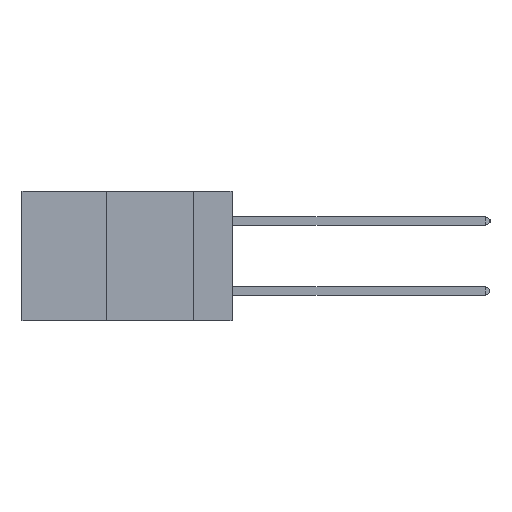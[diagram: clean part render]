
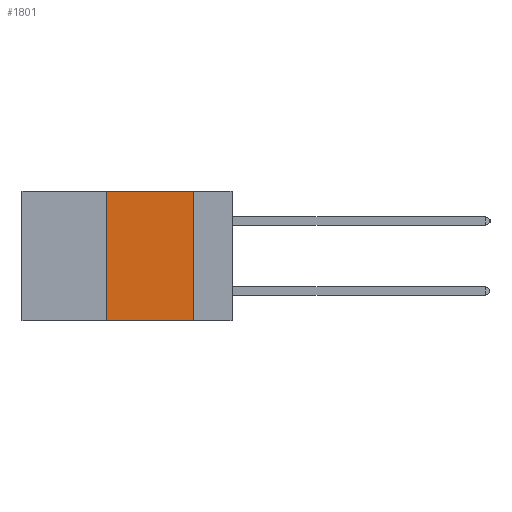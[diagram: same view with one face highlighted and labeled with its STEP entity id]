
A CAD part, left-side view. The second image highlights one B-rep face of the part: STEP entity #1801.
In plain terms, the highlighted planar face has unit normal (-1, 0, 0).
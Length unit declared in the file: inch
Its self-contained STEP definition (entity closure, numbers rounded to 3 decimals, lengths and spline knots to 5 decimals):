
#631 = EDGE_CURVE ( 'NONE', #7029, #7273, #1548, .T. ) ;
#1147 = EDGE_CURVE ( 'NONE', #3780, #7273, #8352, .T. ) ;
#1320 = PLANE ( 'NONE',  #10939 ) ;
#1548 = LINE ( 'NONE', #11987, #9646 ) ;
#1607 = DIRECTION ( 'NONE',  ( 0., 0., 1. ) ) ;
#1782 = EDGE_CURVE ( 'NONE', #8764, #7029, #9109, .T. ) ;
#1801 = ADVANCED_FACE ( 'NONE', ( #8179 ), #1320, .F. ) ;
#1903 = DIRECTION ( 'NONE',  ( 0., 0., -1. ) ) ;
#2018 = LINE ( 'NONE', #8068, #4219 ) ;
#2099 = CARTESIAN_POINT ( 'NONE',  ( 0., 0.6, 0. ) ) ;
#2986 = ORIENTED_EDGE ( 'NONE', *, *, #631, .F. ) ;
#3023 = ORIENTED_EDGE ( 'NONE', *, *, #1782, .F. ) ;
#3108 = ORIENTED_EDGE ( 'NONE', *, *, #9652, .F. ) ;
#3199 = ORIENTED_EDGE ( 'NONE', *, *, #1147, .T. ) ;
#3687 = CARTESIAN_POINT ( 'NONE',  ( 0., 0.11, -0.37 ) ) ;
#3780 = VERTEX_POINT ( 'NONE', #5218 ) ;
#4219 = VECTOR ( 'NONE', #1607, 39.37008 ) ;
#5218 = CARTESIAN_POINT ( 'NONE',  ( 0., 0.36, -0.37 ) ) ;
#6513 = CARTESIAN_POINT ( 'NONE',  ( 0., 0.11, 0. ) ) ;
#7029 = VERTEX_POINT ( 'NONE', #6513 ) ;
#7273 = VERTEX_POINT ( 'NONE', #3687 ) ;
#8068 = CARTESIAN_POINT ( 'NONE',  ( 0., 0.36, 0. ) ) ;
#8179 = FACE_OUTER_BOUND ( 'NONE', #10351, .T. ) ;
#8352 = LINE ( 'NONE', #10961, #10556 ) ;
#8764 = VERTEX_POINT ( 'NONE', #9500 ) ;
#9109 = LINE ( 'NONE', #2099, #11220 ) ;
#9484 = DIRECTION ( 'NONE',  ( 0., 0., -1. ) ) ;
#9500 = CARTESIAN_POINT ( 'NONE',  ( 0., 0.36, 0. ) ) ;
#9646 = VECTOR ( 'NONE', #1903, 39.37008 ) ;
#9652 = EDGE_CURVE ( 'NONE', #3780, #8764, #2018, .T. ) ;
#10042 = DIRECTION ( 'NONE',  ( 1., 0., 0. ) ) ;
#10073 = DIRECTION ( 'NONE',  ( 0., -1., 0. ) ) ;
#10351 = EDGE_LOOP ( 'NONE', ( #2986, #3023, #3108, #3199 ) ) ;
#10556 = VECTOR ( 'NONE', #12682, 39.37008 ) ;
#10939 = AXIS2_PLACEMENT_3D ( 'NONE', #11748, #10042, #9484 ) ;
#10961 = CARTESIAN_POINT ( 'NONE',  ( 0., 0.6, -0.37 ) ) ;
#11220 = VECTOR ( 'NONE', #10073, 39.37008 ) ;
#11748 = CARTESIAN_POINT ( 'NONE',  ( 0., 0.6, 0. ) ) ;
#11987 = CARTESIAN_POINT ( 'NONE',  ( 0., 0.11, 0. ) ) ;
#12682 = DIRECTION ( 'NONE',  ( 0., -1., 0. ) ) ;
